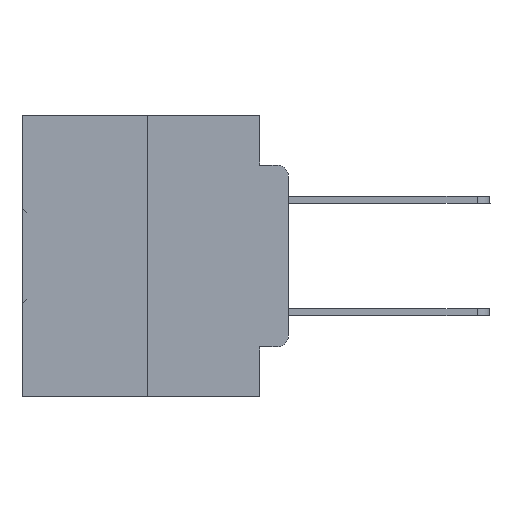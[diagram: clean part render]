
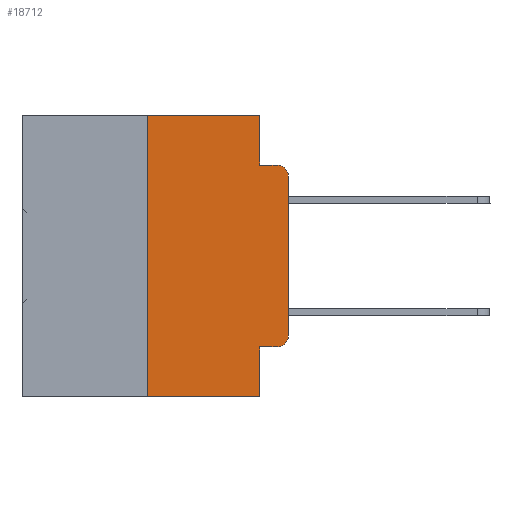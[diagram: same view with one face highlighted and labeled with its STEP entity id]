
A CAD part, left-side view. The second image highlights one B-rep face of the part: STEP entity #18712.
In plain terms, the highlighted planar face has unit normal (-1, 0, 0).
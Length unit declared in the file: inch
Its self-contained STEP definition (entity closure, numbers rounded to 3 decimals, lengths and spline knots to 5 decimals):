
#690 = DIRECTION ( 'NONE',  ( 0., 0., -1. ) ) ;
#1855 = CARTESIAN_POINT ( 'NONE',  ( 0., 0.473, -0.5 ) ) ;
#2744 = CARTESIAN_POINT ( 'NONE',  ( 0., 0.25, -0.5 ) ) ;
#3313 = ORIENTED_EDGE ( 'NONE', *, *, #26754, .T. ) ;
#5450 = AXIS2_PLACEMENT_3D ( 'NONE', #22534, #19423, #14100 ) ;
#6021 = LINE ( 'NONE', #6083, #25268 ) ;
#6083 = CARTESIAN_POINT ( 'NONE',  ( 0., 0.051, 0. ) ) ;
#6090 = ORIENTED_EDGE ( 'NONE', *, *, #30149, .T. ) ;
#6503 = ORIENTED_EDGE ( 'NONE', *, *, #25973, .F. ) ;
#6715 = ORIENTED_EDGE ( 'NONE', *, *, #30412, .F. ) ;
#7194 = CARTESIAN_POINT ( 'NONE',  ( 0., 0.051, -0.0885 ) ) ;
#7362 = DIRECTION ( 'NONE',  ( 0., -1., 0. ) ) ;
#8233 = VECTOR ( 'NONE', #32667, 39.37008 ) ;
#8567 = VERTEX_POINT ( 'NONE', #30787 ) ;
#8909 = EDGE_CURVE ( 'NONE', #33146, #24302, #6021, .T. ) ;
#9179 = LINE ( 'NONE', #18025, #14725 ) ;
#9275 = CARTESIAN_POINT ( 'NONE',  ( 0., 0.02, -0.3915 ) ) ;
#9954 = CARTESIAN_POINT ( 'NONE',  ( 0., 0.02, -0.4115 ) ) ;
#10447 = EDGE_CURVE ( 'NONE', #31660, #27394, #12028, .T. ) ;
#10615 = CARTESIAN_POINT ( 'NONE',  ( 0., 0.25, 0. ) ) ;
#12028 = LINE ( 'NONE', #1855, #23994 ) ;
#12164 = DIRECTION ( 'NONE',  ( 0., 0., -1. ) ) ;
#12825 = LINE ( 'NONE', #10615, #26493 ) ;
#14100 = DIRECTION ( 'NONE',  ( 0., 0., -1. ) ) ;
#14171 = CARTESIAN_POINT ( 'NONE',  ( 0., 0.473, 0. ) ) ;
#14470 = LINE ( 'NONE', #23611, #29879 ) ;
#14725 = VECTOR ( 'NONE', #20757, 39.37008 ) ;
#16117 = CIRCLE ( 'NONE', #5450, 0.02 ) ;
#16306 = DIRECTION ( 'NONE',  ( 0., 0., 1. ) ) ;
#16359 = LINE ( 'NONE', #24531, #8233 ) ;
#16540 = VERTEX_POINT ( 'NONE', #22638 ) ;
#16604 = VERTEX_POINT ( 'NONE', #25759 ) ;
#16978 = DIRECTION ( 'NONE',  ( 0., -1., 0. ) ) ;
#17124 = PLANE ( 'NONE',  #30456 ) ;
#17401 = FACE_OUTER_BOUND ( 'NONE', #29643, .T. ) ;
#17915 = ORIENTED_EDGE ( 'NONE', *, *, #34847, .T. ) ;
#18025 = CARTESIAN_POINT ( 'NONE',  ( 0., 0.051, 0. ) ) ;
#18712 = ADVANCED_FACE ( 'NONE', ( #17401 ), #17124, .F. ) ;
#19423 = DIRECTION ( 'NONE',  ( -1., 0., 0. ) ) ;
#19590 = CARTESIAN_POINT ( 'NONE',  ( 0., 0.473, 0. ) ) ;
#19691 = CARTESIAN_POINT ( 'NONE',  ( 0., 0.051, 0. ) ) ;
#20421 = ORIENTED_EDGE ( 'NONE', *, *, #10447, .T. ) ;
#20546 = VERTEX_POINT ( 'NONE', #32042 ) ;
#20757 = DIRECTION ( 'NONE',  ( 0., 0., -1. ) ) ;
#22534 = CARTESIAN_POINT ( 'NONE',  ( 0., 0.02, -0.1085 ) ) ;
#22638 = CARTESIAN_POINT ( 'NONE',  ( 0., 0., -0.1085 ) ) ;
#23054 = LINE ( 'NONE', #19590, #24805 ) ;
#23611 = CARTESIAN_POINT ( 'NONE',  ( 0., 0.051, -0.4115 ) ) ;
#23725 = DIRECTION ( 'NONE',  ( 0., -1., 0. ) ) ;
#23994 = VECTOR ( 'NONE', #23725, 39.37008 ) ;
#24302 = VERTEX_POINT ( 'NONE', #7194 ) ;
#24377 = EDGE_CURVE ( 'NONE', #24302, #16604, #31318, .T. ) ;
#24531 = CARTESIAN_POINT ( 'NONE',  ( 0., 0., 0. ) ) ;
#24805 = VECTOR ( 'NONE', #16978, 39.37008 ) ;
#24909 = ORIENTED_EDGE ( 'NONE', *, *, #29639, .F. ) ;
#25157 = DIRECTION ( 'NONE',  ( 1., 0., 0. ) ) ;
#25268 = VECTOR ( 'NONE', #690, 39.37008 ) ;
#25759 = CARTESIAN_POINT ( 'NONE',  ( 0., 0.02, -0.0885 ) ) ;
#25973 = EDGE_CURVE ( 'NONE', #8567, #33146, #23054, .T. ) ;
#26018 = DIRECTION ( 'NONE',  ( -1., 0., 0. ) ) ;
#26493 = VECTOR ( 'NONE', #16306, 39.37008 ) ;
#26532 = CIRCLE ( 'NONE', #30385, 0.02 ) ;
#26754 = EDGE_CURVE ( 'NONE', #33727, #32676, #14470, .T. ) ;
#27394 = VERTEX_POINT ( 'NONE', #31451 ) ;
#29167 = DIRECTION ( 'NONE',  ( 0., -1., 0. ) ) ;
#29639 = EDGE_CURVE ( 'NONE', #33727, #27394, #9179, .T. ) ;
#29643 = EDGE_LOOP ( 'NONE', ( #17915, #30663, #31721, #33195, #6503, #6715, #20421, #24909, #3313, #6090 ) ) ;
#29879 = VECTOR ( 'NONE', #7362, 39.37008 ) ;
#30149 = EDGE_CURVE ( 'NONE', #32676, #20546, #26532, .T. ) ;
#30385 = AXIS2_PLACEMENT_3D ( 'NONE', #9275, #26018, #12164 ) ;
#30412 = EDGE_CURVE ( 'NONE', #31660, #8567, #12825, .T. ) ;
#30456 = AXIS2_PLACEMENT_3D ( 'NONE', #14171, #25157, #33669 ) ;
#30476 = VECTOR ( 'NONE', #29167, 39.37008 ) ;
#30663 = ORIENTED_EDGE ( 'NONE', *, *, #31769, .T. ) ;
#30787 = CARTESIAN_POINT ( 'NONE',  ( 0., 0.25, 0. ) ) ;
#31318 = LINE ( 'NONE', #32061, #30476 ) ;
#31451 = CARTESIAN_POINT ( 'NONE',  ( 0., 0.051, -0.5 ) ) ;
#31660 = VERTEX_POINT ( 'NONE', #2744 ) ;
#31721 = ORIENTED_EDGE ( 'NONE', *, *, #24377, .F. ) ;
#31769 = EDGE_CURVE ( 'NONE', #16540, #16604, #16117, .T. ) ;
#32042 = CARTESIAN_POINT ( 'NONE',  ( 0., 0., -0.3915 ) ) ;
#32061 = CARTESIAN_POINT ( 'NONE',  ( 0., 0.051, -0.0885 ) ) ;
#32667 = DIRECTION ( 'NONE',  ( 0., 0., 1. ) ) ;
#32676 = VERTEX_POINT ( 'NONE', #9954 ) ;
#32859 = CARTESIAN_POINT ( 'NONE',  ( 0., 0.051, -0.4115 ) ) ;
#33146 = VERTEX_POINT ( 'NONE', #19691 ) ;
#33195 = ORIENTED_EDGE ( 'NONE', *, *, #8909, .F. ) ;
#33669 = DIRECTION ( 'NONE',  ( 0., 0., -1. ) ) ;
#33727 = VERTEX_POINT ( 'NONE', #32859 ) ;
#34847 = EDGE_CURVE ( 'NONE', #20546, #16540, #16359, .T. ) ;
